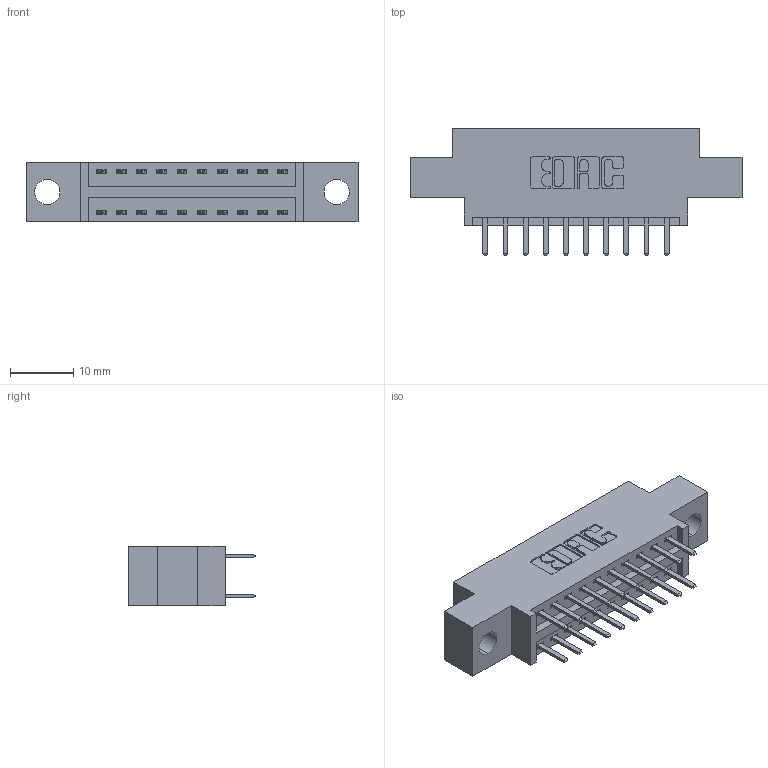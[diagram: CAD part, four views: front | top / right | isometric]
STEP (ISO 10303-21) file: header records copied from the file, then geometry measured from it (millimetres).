
FILE_DESCRIPTION (( 'STEP AP203' ), '1' );
FILE_NAME ('346-020-520-804.STEP', '2022-05-18T18:43:35', ( '' ), ( '' ), 'SwSTEP 2.0', 'SolidWorks 2020', '' );
FILE_SCHEMA (( 'CONFIG_CONTROL_DESIGN' ));
Length unit declared in the file: inch
Products named in the file (3): 346 Part_0.170 Offset - 0.156 Dia-TH; 345-292-001_345-293-120; 346-020-520-804
Assembly tree (21 placements, depth 2):
  346-020-520-804
    346 Part_0.170 Offset - 0.156 Dia-TH
    345-292-001_345-293-120  x20
Bounding box: 52.32 x 20.02 x 9.4 mm (x, y, z)
Volume: 4584.3 mm3; surface area: 5805.4 mm2
Topology: 21 solids, 21 shells, 1260 faces, 3637 edges, 2370 vertices
Faces by surface type: plane 834, cylinder 426
Entity records: 11499 total; most frequent: CARTESIAN_POINT 1958, ORIENTED_EDGE 1878, DIRECTION 1763, EDGE_CURVE 939, VECTOR 763, LINE 763, VERTEX_POINT 622, AXIS2_PLACEMENT_3D 500
